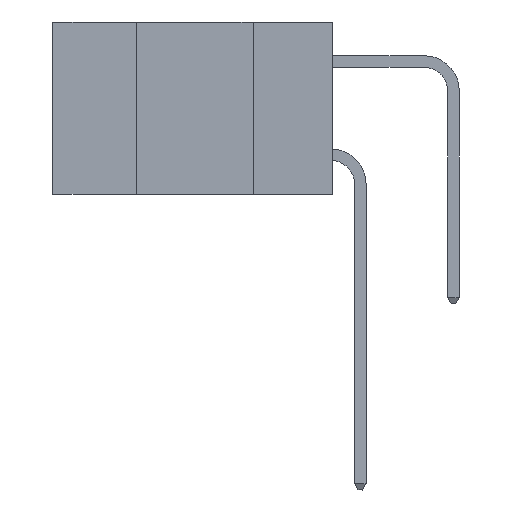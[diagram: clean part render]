
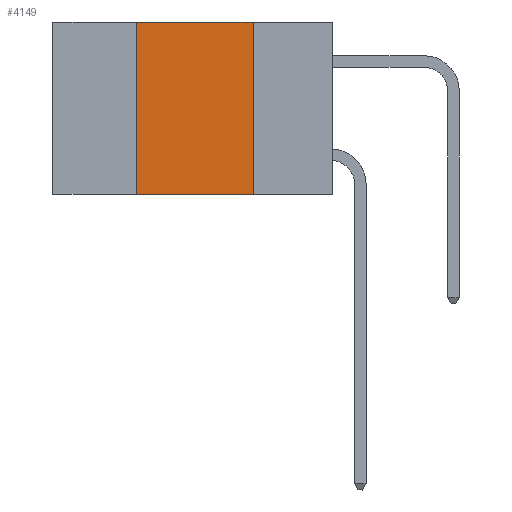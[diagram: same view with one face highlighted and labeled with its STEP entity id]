
A CAD part, left-side view. The second image highlights one B-rep face of the part: STEP entity #4149.
In plain terms, the highlighted planar face has unit normal (-1, 0, 0).
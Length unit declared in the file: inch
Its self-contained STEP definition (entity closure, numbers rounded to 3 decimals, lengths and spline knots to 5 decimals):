
#94 = EDGE_LOOP ( 'NONE', ( #6163, #4038, #1613, #4611 ) ) ;
#169 = DIRECTION ( 'NONE',  ( 0., 0., 1. ) ) ;
#684 = VECTOR ( 'NONE', #10232, 39.37008 ) ;
#703 = DIRECTION ( 'NONE',  ( 0., -1., 0. ) ) ;
#854 = PLANE ( 'NONE',  #6704 ) ;
#879 = VERTEX_POINT ( 'NONE', #2265 ) ;
#1613 = ORIENTED_EDGE ( 'NONE', *, *, #7671, .F. ) ;
#1771 = DIRECTION ( 'NONE',  ( 1., 0., 0. ) ) ;
#1996 = DIRECTION ( 'NONE',  ( 0., 0., -1. ) ) ;
#2080 = EDGE_CURVE ( 'NONE', #11503, #879, #10885, .T. ) ;
#2265 = CARTESIAN_POINT ( 'NONE',  ( 0., 0.17, -0.37 ) ) ;
#2651 = VERTEX_POINT ( 'NONE', #8761 ) ;
#3344 = LINE ( 'NONE', #9782, #10346 ) ;
#4038 = ORIENTED_EDGE ( 'NONE', *, *, #11308, .F. ) ;
#4149 = ADVANCED_FACE ( 'NONE', ( #7540 ), #854, .F. ) ;
#4611 = ORIENTED_EDGE ( 'NONE', *, *, #2080, .T. ) ;
#5267 = CARTESIAN_POINT ( 'NONE',  ( 0., 0.42, 0. ) ) ;
#5621 = CARTESIAN_POINT ( 'NONE',  ( 0., 0.6, 0. ) ) ;
#6163 = ORIENTED_EDGE ( 'NONE', *, *, #7872, .F. ) ;
#6704 = AXIS2_PLACEMENT_3D ( 'NONE', #8910, #1771, #1996 ) ;
#7233 = LINE ( 'NONE', #5267, #11858 ) ;
#7540 = FACE_OUTER_BOUND ( 'NONE', #94, .T. ) ;
#7671 = EDGE_CURVE ( 'NONE', #11503, #9963, #7233, .T. ) ;
#7872 = EDGE_CURVE ( 'NONE', #2651, #879, #3344, .T. ) ;
#7947 = LINE ( 'NONE', #5621, #9783 ) ;
#8761 = CARTESIAN_POINT ( 'NONE',  ( 0., 0.17, 0. ) ) ;
#8910 = CARTESIAN_POINT ( 'NONE',  ( 0., 0.6, 0. ) ) ;
#9437 = CARTESIAN_POINT ( 'NONE',  ( 0., 0.42, -0.37 ) ) ;
#9630 = CARTESIAN_POINT ( 'NONE',  ( 0., 0.42, 0. ) ) ;
#9782 = CARTESIAN_POINT ( 'NONE',  ( 0., 0.17, 0. ) ) ;
#9783 = VECTOR ( 'NONE', #703, 39.37008 ) ;
#9830 = DIRECTION ( 'NONE',  ( 0., 0., -1. ) ) ;
#9963 = VERTEX_POINT ( 'NONE', #9630 ) ;
#10232 = DIRECTION ( 'NONE',  ( 0., -1., 0. ) ) ;
#10346 = VECTOR ( 'NONE', #9830, 39.37008 ) ;
#10885 = LINE ( 'NONE', #11693, #684 ) ;
#11308 = EDGE_CURVE ( 'NONE', #9963, #2651, #7947, .T. ) ;
#11503 = VERTEX_POINT ( 'NONE', #9437 ) ;
#11693 = CARTESIAN_POINT ( 'NONE',  ( 0., 0.6, -0.37 ) ) ;
#11858 = VECTOR ( 'NONE', #169, 39.37008 ) ;
